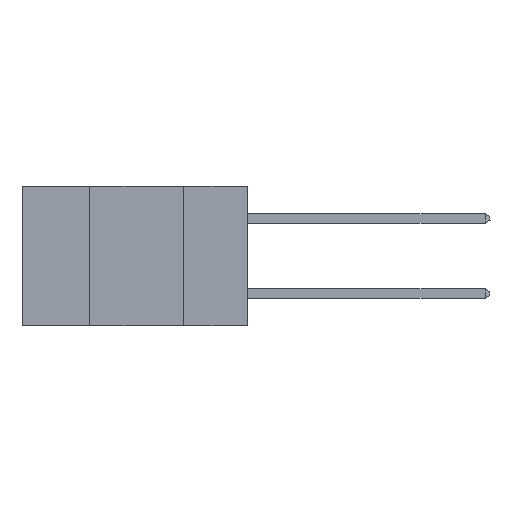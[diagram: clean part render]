
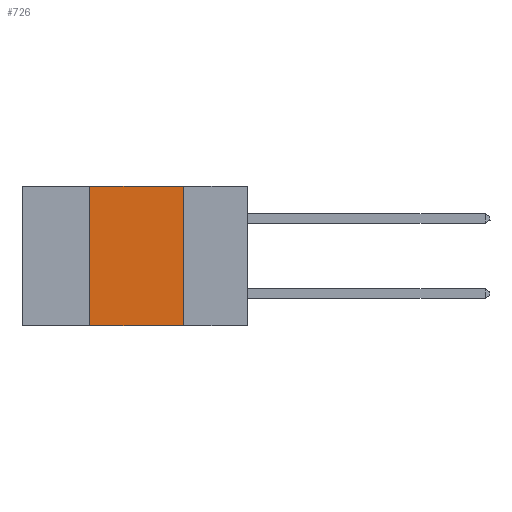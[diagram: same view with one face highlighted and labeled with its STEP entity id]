
A CAD part, left-side view. The second image highlights one B-rep face of the part: STEP entity #726.
In plain terms, the highlighted planar face has unit normal (-1, 0, 0).
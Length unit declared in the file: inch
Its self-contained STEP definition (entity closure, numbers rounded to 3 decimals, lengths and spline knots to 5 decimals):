
#726 = ADVANCED_FACE ( 'NONE', ( #14484 ), #23607, .F. ) ;
#2493 = CARTESIAN_POINT ( 'NONE',  ( 0., 0.6, -0.37 ) ) ;
#2840 = DIRECTION ( 'NONE',  ( 1., 0., 0. ) ) ;
#3715 = VECTOR ( 'NONE', #12217, 39.37008 ) ;
#5470 = EDGE_CURVE ( 'NONE', #11792, #17800, #23157, .T. ) ;
#5512 = LINE ( 'NONE', #2493, #19027 ) ;
#5697 = DIRECTION ( 'NONE',  ( 0., 0., -1. ) ) ;
#6802 = DIRECTION ( 'NONE',  ( 0., 0., -1. ) ) ;
#7462 = VERTEX_POINT ( 'NONE', #8219 ) ;
#8219 = CARTESIAN_POINT ( 'NONE',  ( 0., 0.42, -0.37 ) ) ;
#8368 = DIRECTION ( 'NONE',  ( 0., 0., 1. ) ) ;
#8533 = LINE ( 'NONE', #17830, #23004 ) ;
#9324 = VECTOR ( 'NONE', #8368, 39.37008 ) ;
#9895 = CARTESIAN_POINT ( 'NONE',  ( 0., 0.17, -0.37 ) ) ;
#11401 = EDGE_LOOP ( 'NONE', ( #11425, #13417, #14477, #23731 ) ) ;
#11425 = ORIENTED_EDGE ( 'NONE', *, *, #12509, .F. ) ;
#11792 = VERTEX_POINT ( 'NONE', #15904 ) ;
#12217 = DIRECTION ( 'NONE',  ( 0., -1., 0. ) ) ;
#12509 = EDGE_CURVE ( 'NONE', #17800, #21201, #8533, .T. ) ;
#13417 = ORIENTED_EDGE ( 'NONE', *, *, #5470, .F. ) ;
#13672 = DIRECTION ( 'NONE',  ( 0., -1., 0. ) ) ;
#14477 = ORIENTED_EDGE ( 'NONE', *, *, #23030, .F. ) ;
#14484 = FACE_OUTER_BOUND ( 'NONE', #11401, .T. ) ;
#15904 = CARTESIAN_POINT ( 'NONE',  ( 0., 0.42, 0. ) ) ;
#17075 = EDGE_CURVE ( 'NONE', #7462, #21201, #5512, .T. ) ;
#17538 = CARTESIAN_POINT ( 'NONE',  ( 0., 0.42, -0.37 ) ) ;
#17800 = VERTEX_POINT ( 'NONE', #19142 ) ;
#17830 = CARTESIAN_POINT ( 'NONE',  ( 0., 0.17, -0.37 ) ) ;
#18035 = AXIS2_PLACEMENT_3D ( 'NONE', #23689, #2840, #5697 ) ;
#19027 = VECTOR ( 'NONE', #13672, 39.37008 ) ;
#19142 = CARTESIAN_POINT ( 'NONE',  ( 0., 0.17, 0. ) ) ;
#19416 = CARTESIAN_POINT ( 'NONE',  ( 0., 0.6, 0. ) ) ;
#21201 = VERTEX_POINT ( 'NONE', #9895 ) ;
#23004 = VECTOR ( 'NONE', #6802, 39.37008 ) ;
#23030 = EDGE_CURVE ( 'NONE', #7462, #11792, #23233, .T. ) ;
#23157 = LINE ( 'NONE', #19416, #3715 ) ;
#23233 = LINE ( 'NONE', #17538, #9324 ) ;
#23607 = PLANE ( 'NONE',  #18035 ) ;
#23689 = CARTESIAN_POINT ( 'NONE',  ( 0., 0.6, 0. ) ) ;
#23731 = ORIENTED_EDGE ( 'NONE', *, *, #17075, .T. ) ;
